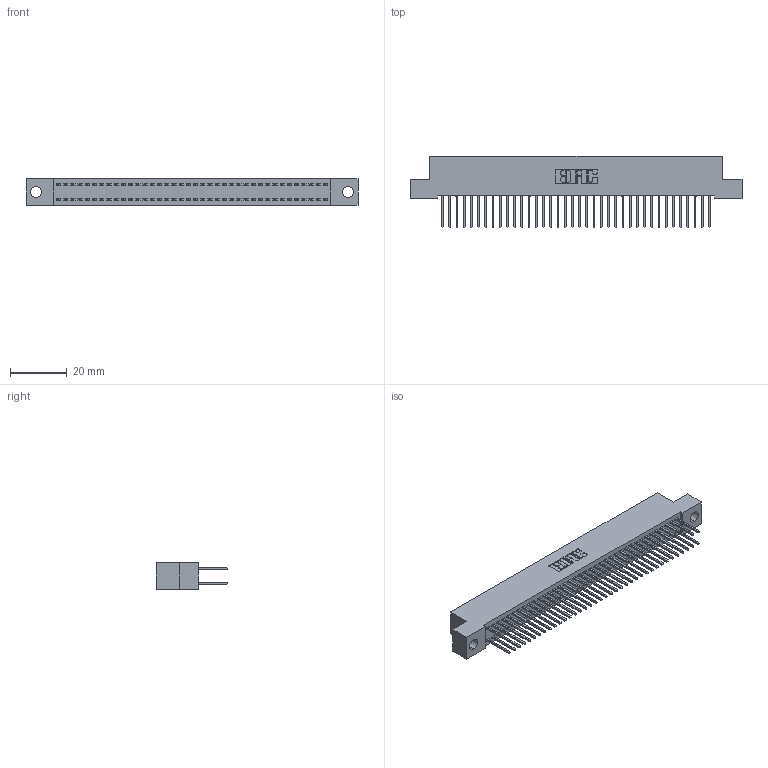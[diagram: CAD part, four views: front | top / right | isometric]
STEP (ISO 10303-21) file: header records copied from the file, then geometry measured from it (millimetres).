
FILE_DESCRIPTION (( 'STEP AP203' ), '1' );
FILE_NAME ('342-076-523-204.STEP', '2019-10-04T10:38:49', ( '' ), ( '' ), 'SwSTEP 2.0', 'SolidWorks 2016', '' );
FILE_SCHEMA (( 'CONFIG_CONTROL_DESIGN' ));
Length unit declared in the file: inch
Products named in the file (3): 345-292-001_345-293-123; 342-076-523-204; 342 Part_.156 TH
Assembly tree (77 placements, depth 2):
  342-076-523-204
    342 Part_.156 TH
    345-292-001_345-293-123  x76
Bounding box: 116.84 x 25.15 x 9.4 mm (x, y, z)
Volume: 10547.9 mm3; surface area: 17557.6 mm2
Topology: 77 solids, 77 shells, 4062 faces, 12079 edges, 7950 vertices
Faces by surface type: plane 2802, cylinder 1260
Entity records: 24853 total; most frequent: CARTESIAN_POINT 4122, ORIENTED_EDGE 4058, DIRECTION 3529, EDGE_CURVE 2029, LINE 1901, VECTOR 1901, VERTEX_POINT 1350, AXIS2_PLACEMENT_3D 814
